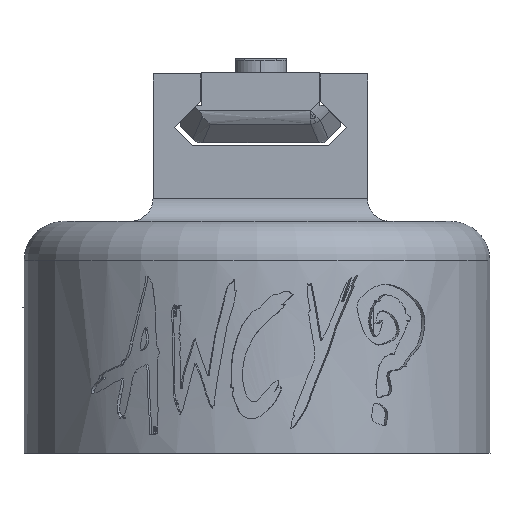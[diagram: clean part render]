
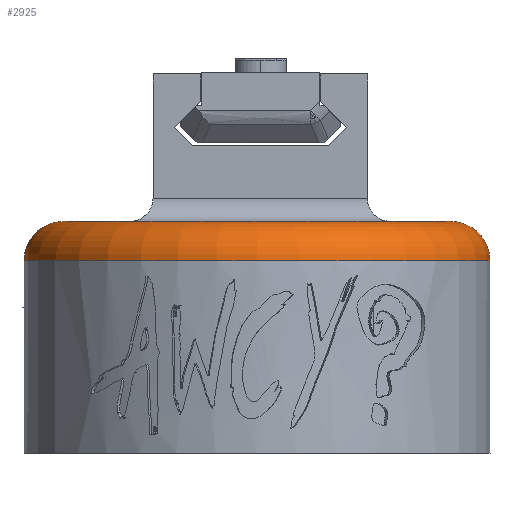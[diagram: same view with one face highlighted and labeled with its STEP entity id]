
A CAD part, front view. The second image highlights one B-rep face of the part: STEP entity #2925.
In plain terms, the highlighted toroidal (fillet/blend) face has major radius 25.57 mm and minor radius 5.18 mm.
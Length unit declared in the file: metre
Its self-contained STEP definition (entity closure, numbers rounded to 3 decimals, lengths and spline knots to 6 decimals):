
#2925=ADVANCED_FACE('0:6013',(#6420,#6421),#6422,.T.);
#6420=FACE_BOUND('',#26078,.T.);
#6421=FACE_BOUND('',#26079,.T.);
#6422=TOROIDAL_SURFACE('',#26080,0.02557,0.00518);
#26078=EDGE_LOOP('',(#49174,#49175));
#26079=EDGE_LOOP('',(#49176,#49177));
#26080=AXIS2_PLACEMENT_3D('',#49178,#49179,#49180);
#49174=ORIENTED_EDGE('',*,*,#61861,.T.);
#49175=ORIENTED_EDGE('',*,*,#61862,.T.);
#49176=ORIENTED_EDGE('',*,*,#63692,.F.);
#49177=ORIENTED_EDGE('',*,*,#63693,.F.);
#49178=CARTESIAN_POINT('',(-0.0452,0.03997,0.00414));
#49179=DIRECTION('',(0.0,0.,-1.0));
#49180=DIRECTION('',(-1.0,0.0,0.0));
#61861=EDGE_CURVE('0:20337',#84875,#84876,#84877,.T.);
#61862=EDGE_CURVE('0:20337',#84876,#84875,#84878,.T.);
#63692=EDGE_CURVE('0:20334',#87631,#87632,#87633,.T.);
#63693=EDGE_CURVE('0:20334',#87632,#87631,#87634,.T.);
#84875=VERTEX_POINT('',#105704);
#84876=VERTEX_POINT('',#105705);
#84877=CIRCLE('',#105706,0.02557);
#84878=CIRCLE('',#105707,0.02557);
#87631=VERTEX_POINT('',#117999);
#87632=VERTEX_POINT('',#118000);
#87633=CIRCLE('',#118001,0.03075);
#87634=CIRCLE('',#118002,0.03075);
#105704=CARTESIAN_POINT('',(-0.07077,0.03997,-0.00104));
#105705=CARTESIAN_POINT('',(-0.01963,0.03997,-0.00104));
#105706=AXIS2_PLACEMENT_3D('',#133712,#133713,#133714);
#105707=AXIS2_PLACEMENT_3D('',#133715,#133716,#133717);
#117999=CARTESIAN_POINT('',(-0.02979,0.06658,0.00414));
#118000=CARTESIAN_POINT('',(-0.06061,0.01336,0.00414));
#118001=AXIS2_PLACEMENT_3D('',#134583,#134584,#134585);
#118002=AXIS2_PLACEMENT_3D('',#134586,#134587,#134588);
#133712=CARTESIAN_POINT('',(-0.0452,0.03997,-0.00104));
#133713=DIRECTION('',(0.,0.,1.0));
#133714=DIRECTION('',(1.0,0.,0.));
#133715=CARTESIAN_POINT('',(-0.0452,0.03997,-0.00104));
#133716=DIRECTION('',(0.,0.,1.0));
#133717=DIRECTION('',(1.0,0.,0.));
#134583=CARTESIAN_POINT('',(-0.0452,0.03997,0.00414));
#134584=DIRECTION('',(0.,0.,1.0));
#134585=DIRECTION('',(1.0,0.,0.));
#134586=CARTESIAN_POINT('',(-0.0452,0.03997,0.00414));
#134587=DIRECTION('',(0.,0.,1.0));
#134588=DIRECTION('',(1.0,0.,0.));
